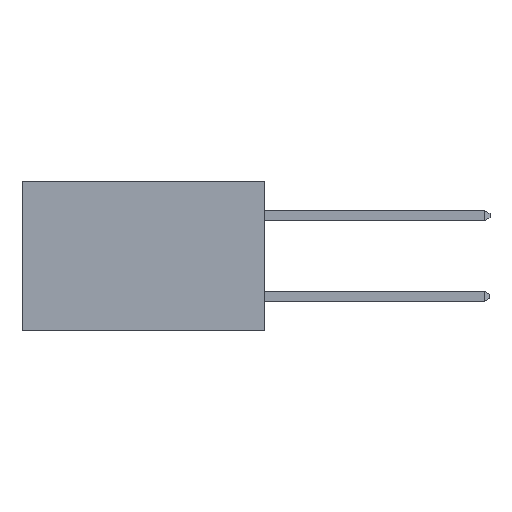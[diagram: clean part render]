
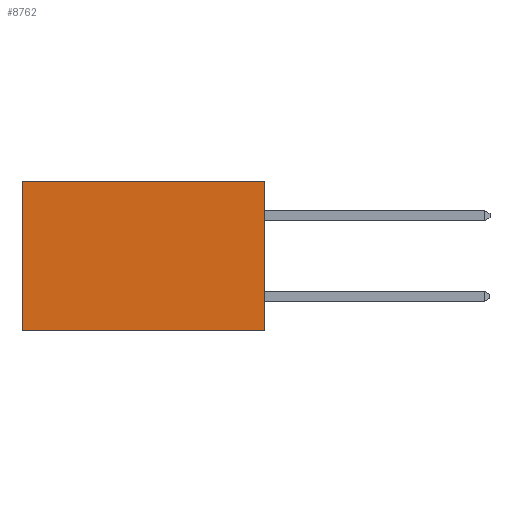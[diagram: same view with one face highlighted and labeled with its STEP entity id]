
A CAD part, left-side view. The second image highlights one B-rep face of the part: STEP entity #8762.
In plain terms, the highlighted planar face has unit normal (-1, 0, 0).
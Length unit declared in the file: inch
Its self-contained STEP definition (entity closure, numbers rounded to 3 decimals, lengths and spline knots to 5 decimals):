
#36 = DIRECTION ( 'NONE',  ( 0., 0., -1. ) ) ;
#317 = DIRECTION ( 'NONE',  ( 1., 0., 0. ) ) ;
#734 = VECTOR ( 'NONE', #2436, 39.37008 ) ;
#1369 = EDGE_CURVE ( 'NONE', #6501, #3201, #4130, .T. ) ;
#1528 = DIRECTION ( 'NONE',  ( 0., 0., -1. ) ) ;
#1571 = ORIENTED_EDGE ( 'NONE', *, *, #1369, .F. ) ;
#1684 = LINE ( 'NONE', #3270, #734 ) ;
#1913 = VERTEX_POINT ( 'NONE', #5848 ) ;
#2136 = VECTOR ( 'NONE', #8833, 39.37008 ) ;
#2436 = DIRECTION ( 'NONE',  ( 0., 1., 0. ) ) ;
#2806 = ORIENTED_EDGE ( 'NONE', *, *, #3421, .F. ) ;
#3033 = LINE ( 'NONE', #7591, #4684 ) ;
#3201 = VERTEX_POINT ( 'NONE', #5805 ) ;
#3270 = CARTESIAN_POINT ( 'NONE',  ( 0.2615, 0., 0. ) ) ;
#3380 = CARTESIAN_POINT ( 'NONE',  ( 0.2615, 0., -0.37 ) ) ;
#3421 = EDGE_CURVE ( 'NONE', #3901, #6501, #4514, .T. ) ;
#3901 = VERTEX_POINT ( 'NONE', #7860 ) ;
#4130 = LINE ( 'NONE', #3380, #2136 ) ;
#4396 = AXIS2_PLACEMENT_3D ( 'NONE', #7720, #317, #1528 ) ;
#4507 = EDGE_LOOP ( 'NONE', ( #7131, #1571, #2806, #9012 ) ) ;
#4514 = LINE ( 'NONE', #6760, #9402 ) ;
#4684 = VECTOR ( 'NONE', #36, 39.37008 ) ;
#5805 = CARTESIAN_POINT ( 'NONE',  ( 0.2615, 0.6, -0.37 ) ) ;
#5848 = CARTESIAN_POINT ( 'NONE',  ( 0.2615, 0.6, 0. ) ) ;
#6389 = FACE_OUTER_BOUND ( 'NONE', #4507, .T. ) ;
#6501 = VERTEX_POINT ( 'NONE', #8676 ) ;
#6760 = CARTESIAN_POINT ( 'NONE',  ( 0.2615, 0., -0.37 ) ) ;
#7131 = ORIENTED_EDGE ( 'NONE', *, *, #7385, .T. ) ;
#7385 = EDGE_CURVE ( 'NONE', #1913, #3201, #3033, .T. ) ;
#7591 = CARTESIAN_POINT ( 'NONE',  ( 0.2615, 0.6, -0.37 ) ) ;
#7660 = PLANE ( 'NONE',  #4396 ) ;
#7720 = CARTESIAN_POINT ( 'NONE',  ( 0.2615, 0., -0.37 ) ) ;
#7860 = CARTESIAN_POINT ( 'NONE',  ( 0.2615, 0., 0. ) ) ;
#8441 = EDGE_CURVE ( 'NONE', #3901, #1913, #1684, .T. ) ;
#8676 = CARTESIAN_POINT ( 'NONE',  ( 0.2615, 0., -0.37 ) ) ;
#8762 = ADVANCED_FACE ( 'NONE', ( #6389 ), #7660, .F. ) ;
#8833 = DIRECTION ( 'NONE',  ( 0., 1., 0. ) ) ;
#9012 = ORIENTED_EDGE ( 'NONE', *, *, #8441, .T. ) ;
#9402 = VECTOR ( 'NONE', #9778, 39.37008 ) ;
#9778 = DIRECTION ( 'NONE',  ( 0., 0., -1. ) ) ;
